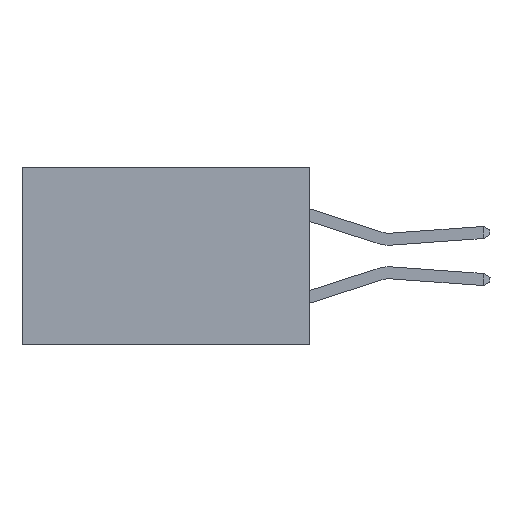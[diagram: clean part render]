
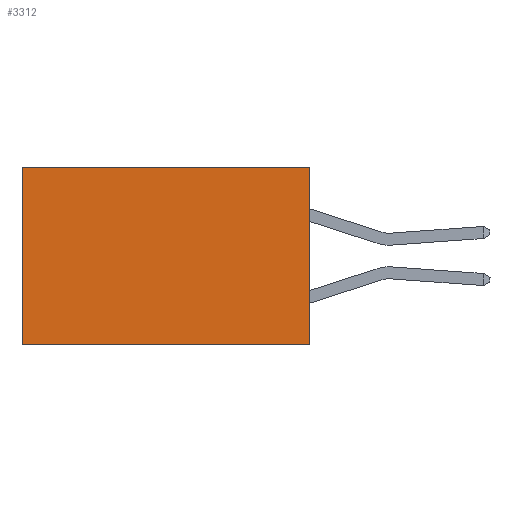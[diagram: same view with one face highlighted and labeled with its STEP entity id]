
A CAD part, left-side view. The second image highlights one B-rep face of the part: STEP entity #3312.
In plain terms, the highlighted planar face has unit normal (-1, 0, 0).
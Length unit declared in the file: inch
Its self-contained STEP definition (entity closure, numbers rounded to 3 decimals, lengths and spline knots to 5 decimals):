
#342 = DIRECTION ( 'NONE',  ( 0., 0., -1. ) ) ;
#427 = LINE ( 'NONE', #2099, #8909 ) ;
#531 = LINE ( 'NONE', #11982, #6491 ) ;
#560 = DIRECTION ( 'NONE',  ( 0., 1., 0. ) ) ;
#1499 = CARTESIAN_POINT ( 'NONE',  ( 0.298, 0.6, 0. ) ) ;
#1618 = ORIENTED_EDGE ( 'NONE', *, *, #9795, .F. ) ;
#2099 = CARTESIAN_POINT ( 'NONE',  ( 0.298, 0., 0. ) ) ;
#3312 = ADVANCED_FACE ( 'NONE', ( #13436 ), #3925, .F. ) ;
#3382 = VERTEX_POINT ( 'NONE', #14387 ) ;
#3925 = PLANE ( 'NONE',  #4641 ) ;
#4266 = EDGE_CURVE ( 'NONE', #12964, #13024, #9166, .T. ) ;
#4479 = DIRECTION ( 'NONE',  ( 0., 0., -1. ) ) ;
#4641 = AXIS2_PLACEMENT_3D ( 'NONE', #12005, #13151, #342 ) ;
#6108 = VECTOR ( 'NONE', #14144, 39.37008 ) ;
#6491 = VECTOR ( 'NONE', #560, 39.37008 ) ;
#6940 = CARTESIAN_POINT ( 'NONE',  ( 0.298, 0., 0. ) ) ;
#7404 = ORIENTED_EDGE ( 'NONE', *, *, #11851, .F. ) ;
#7995 = DIRECTION ( 'NONE',  ( 0., 1., 0. ) ) ;
#8510 = VECTOR ( 'NONE', #7995, 39.37008 ) ;
#8909 = VECTOR ( 'NONE', #4479, 39.37008 ) ;
#9166 = LINE ( 'NONE', #1499, #6108 ) ;
#9367 = ORIENTED_EDGE ( 'NONE', *, *, #4266, .T. ) ;
#9745 = EDGE_LOOP ( 'NONE', ( #9367, #1618, #7404, #14937 ) ) ;
#9795 = EDGE_CURVE ( 'NONE', #3382, #13024, #531, .T. ) ;
#10592 = EDGE_CURVE ( 'NONE', #14718, #12964, #11804, .T. ) ;
#10831 = CARTESIAN_POINT ( 'NONE',  ( 0.298, 0.6, 0. ) ) ;
#11804 = LINE ( 'NONE', #13978, #8510 ) ;
#11851 = EDGE_CURVE ( 'NONE', #14718, #3382, #427, .T. ) ;
#11982 = CARTESIAN_POINT ( 'NONE',  ( 0.298, 0., -0.37 ) ) ;
#12005 = CARTESIAN_POINT ( 'NONE',  ( 0.298, 0., 0. ) ) ;
#12964 = VERTEX_POINT ( 'NONE', #10831 ) ;
#13024 = VERTEX_POINT ( 'NONE', #13569 ) ;
#13151 = DIRECTION ( 'NONE',  ( 1., 0., 0. ) ) ;
#13436 = FACE_OUTER_BOUND ( 'NONE', #9745, .T. ) ;
#13569 = CARTESIAN_POINT ( 'NONE',  ( 0.298, 0.6, -0.37 ) ) ;
#13978 = CARTESIAN_POINT ( 'NONE',  ( 0.298, 0., 0. ) ) ;
#14144 = DIRECTION ( 'NONE',  ( 0., 0., -1. ) ) ;
#14387 = CARTESIAN_POINT ( 'NONE',  ( 0.298, 0., -0.37 ) ) ;
#14718 = VERTEX_POINT ( 'NONE', #6940 ) ;
#14937 = ORIENTED_EDGE ( 'NONE', *, *, #10592, .T. ) ;
